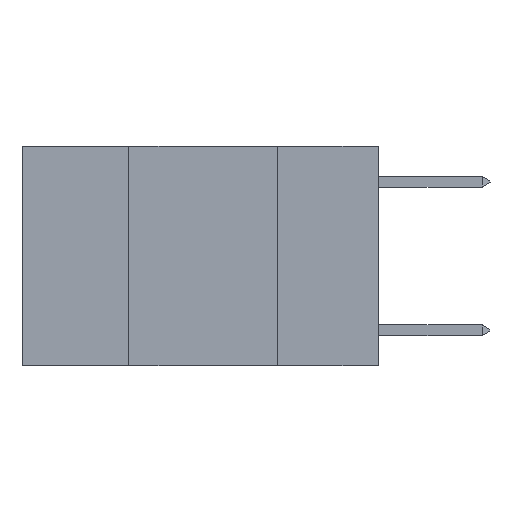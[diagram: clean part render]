
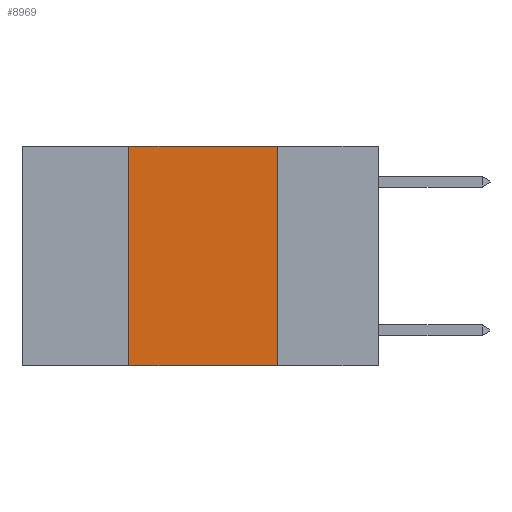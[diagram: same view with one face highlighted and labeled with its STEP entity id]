
A CAD part, left-side view. The second image highlights one B-rep face of the part: STEP entity #8969.
In plain terms, the highlighted planar face has unit normal (-1, 0, 0).
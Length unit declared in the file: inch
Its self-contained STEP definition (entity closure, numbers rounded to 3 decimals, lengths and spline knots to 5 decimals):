
#790 = CARTESIAN_POINT ( 'NONE',  ( 0., 0.17, 0. ) ) ;
#1027 = CARTESIAN_POINT ( 'NONE',  ( 0., 0.42, 0. ) ) ;
#1205 = PLANE ( 'NONE',  #10902 ) ;
#1896 = EDGE_CURVE ( 'NONE', #21511, #3132, #23435, .T. ) ;
#3132 = VERTEX_POINT ( 'NONE', #12616 ) ;
#3453 = DIRECTION ( 'NONE',  ( 0., 0., -1. ) ) ;
#3849 = EDGE_CURVE ( 'NONE', #24654, #12549, #4788, .T. ) ;
#4204 = CARTESIAN_POINT ( 'NONE',  ( 0., 0.6, -0.37 ) ) ;
#4272 = DIRECTION ( 'NONE',  ( 0., -1., 0. ) ) ;
#4788 = LINE ( 'NONE', #4204, #5506 ) ;
#5506 = VECTOR ( 'NONE', #4272, 39.37008 ) ;
#6292 = LINE ( 'NONE', #790, #17279 ) ;
#6575 = ORIENTED_EDGE ( 'NONE', *, *, #16417, .F. ) ;
#6756 = CARTESIAN_POINT ( 'NONE',  ( 0., 0.42, 0. ) ) ;
#7830 = CARTESIAN_POINT ( 'NONE',  ( 0., 0.6, 0. ) ) ;
#8969 = ADVANCED_FACE ( 'NONE', ( #25180 ), #1205, .F. ) ;
#10902 = AXIS2_PLACEMENT_3D ( 'NONE', #7830, #16701, #3453 ) ;
#11712 = EDGE_CURVE ( 'NONE', #24654, #21511, #13553, .T. ) ;
#12549 = VERTEX_POINT ( 'NONE', #16180 ) ;
#12616 = CARTESIAN_POINT ( 'NONE',  ( 0., 0.17, 0. ) ) ;
#13364 = CARTESIAN_POINT ( 'NONE',  ( 0., 0.42, -0.37 ) ) ;
#13553 = LINE ( 'NONE', #6756, #18548 ) ;
#16180 = CARTESIAN_POINT ( 'NONE',  ( 0., 0.17, -0.37 ) ) ;
#16304 = DIRECTION ( 'NONE',  ( 0., 0., -1. ) ) ;
#16417 = EDGE_CURVE ( 'NONE', #3132, #12549, #6292, .T. ) ;
#16643 = ORIENTED_EDGE ( 'NONE', *, *, #1896, .F. ) ;
#16701 = DIRECTION ( 'NONE',  ( 1., 0., 0. ) ) ;
#17279 = VECTOR ( 'NONE', #16304, 39.37008 ) ;
#17681 = DIRECTION ( 'NONE',  ( 0., 0., 1. ) ) ;
#18548 = VECTOR ( 'NONE', #17681, 39.37008 ) ;
#18672 = ORIENTED_EDGE ( 'NONE', *, *, #11712, .F. ) ;
#19654 = ORIENTED_EDGE ( 'NONE', *, *, #3849, .T. ) ;
#21511 = VERTEX_POINT ( 'NONE', #1027 ) ;
#22727 = EDGE_LOOP ( 'NONE', ( #6575, #16643, #18672, #19654 ) ) ;
#22826 = VECTOR ( 'NONE', #24443, 39.37008 ) ;
#23435 = LINE ( 'NONE', #27787, #22826 ) ;
#24443 = DIRECTION ( 'NONE',  ( 0., -1., 0. ) ) ;
#24654 = VERTEX_POINT ( 'NONE', #13364 ) ;
#25180 = FACE_OUTER_BOUND ( 'NONE', #22727, .T. ) ;
#27787 = CARTESIAN_POINT ( 'NONE',  ( 0., 0.6, 0. ) ) ;
